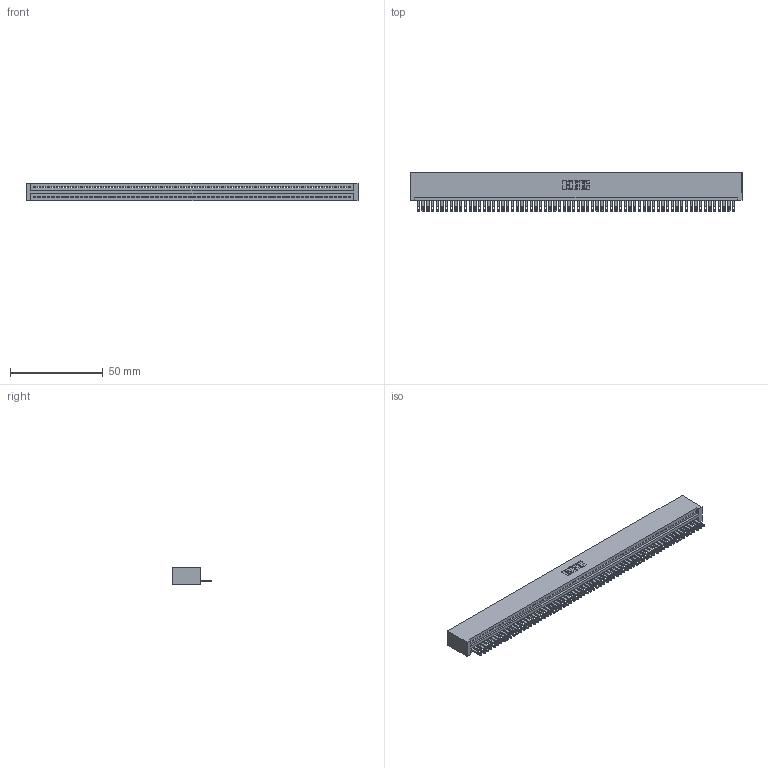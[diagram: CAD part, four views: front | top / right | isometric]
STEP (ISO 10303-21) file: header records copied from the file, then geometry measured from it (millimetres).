
FILE_DESCRIPTION (( 'STEP AP203' ), '1' );
FILE_NAME ('345-068-500-101.STEP', '2018-09-29T05:53:06', ( '' ), ( '' ), 'SwSTEP 2.0', 'SolidWorks 2016', '' );
FILE_SCHEMA (( 'CONFIG_CONTROL_DESIGN' ));
Length unit declared in the file: inch
Products named in the file (3): 345-068-500-101; 345 Part_No Mounting Lugs; 345-292-001_345-293-100
Assembly tree (69 placements, depth 2):
  345-068-500-101
    345 Part_No Mounting Lugs
    345-292-001_345-293-100  x68
Bounding box: 179.32 x 21.51 x 9.4 mm (x, y, z)
Volume: 17871.8 mm3; surface area: 24446.2 mm2
Topology: 69 solids, 69 shells, 3790 faces, 11741 edges, 7826 vertices
Faces by surface type: plane 2388, cylinder 1402
Entity records: 47331 total; most frequent: ORIENTED_EDGE 8206, CARTESIAN_POINT 8204, DIRECTION 7123, EDGE_CURVE 4103, VECTOR 3703, LINE 3703, VERTEX_POINT 2734, AXIS2_PLACEMENT_3D 1710
